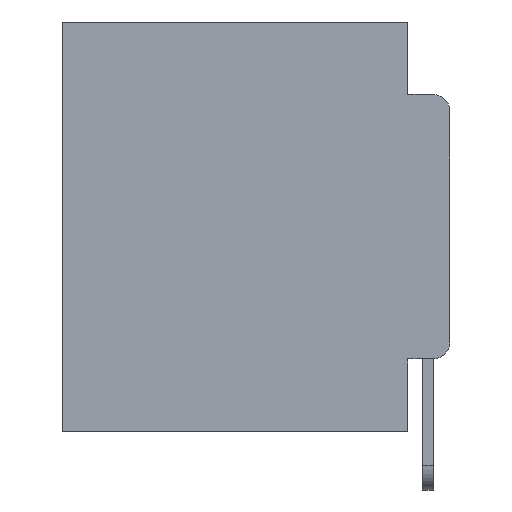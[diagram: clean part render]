
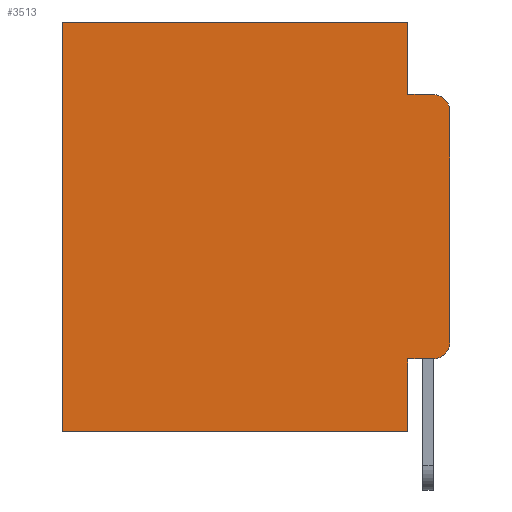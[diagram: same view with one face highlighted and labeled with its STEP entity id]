
A CAD part, left-side view. The second image highlights one B-rep face of the part: STEP entity #3513.
In plain terms, the highlighted planar face has unit normal (-1, 0, 0).
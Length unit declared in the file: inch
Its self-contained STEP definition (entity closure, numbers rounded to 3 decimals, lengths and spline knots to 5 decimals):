
#611 = EDGE_CURVE ( 'NONE', #26364, #8648, #3214, .T. ) ;
#617 = CARTESIAN_POINT ( 'NONE',  ( 0.298, 0., 0. ) ) ;
#1096 = CARTESIAN_POINT ( 'NONE',  ( 0.298, 0.473, 0. ) ) ;
#1326 = CARTESIAN_POINT ( 'NONE',  ( 0.298, 0., -0.1085 ) ) ;
#1452 = ORIENTED_EDGE ( 'NONE', *, *, #611, .F. ) ;
#1643 = CARTESIAN_POINT ( 'NONE',  ( 0.298, 0.051, -0.0885 ) ) ;
#1848 = CARTESIAN_POINT ( 'NONE',  ( 0.298, 0.051, -0.0885 ) ) ;
#2389 = CARTESIAN_POINT ( 'NONE',  ( 0.298, 0.473, 0. ) ) ;
#2427 = VECTOR ( 'NONE', #3080, 39.37008 ) ;
#2431 = DIRECTION ( 'NONE',  ( 0., 0., -1. ) ) ;
#2499 = VECTOR ( 'NONE', #6045, 39.37008 ) ;
#2696 = DIRECTION ( 'NONE',  ( -1., 0., 0. ) ) ;
#2914 = ORIENTED_EDGE ( 'NONE', *, *, #5883, .T. ) ;
#3080 = DIRECTION ( 'NONE',  ( 0., 1., 0. ) ) ;
#3214 = LINE ( 'NONE', #8234, #2499 ) ;
#3513 = ADVANCED_FACE ( 'NONE', ( #10835 ), #6703, .F. ) ;
#3762 = CARTESIAN_POINT ( 'NONE',  ( 0.298, 0.051, 0. ) ) ;
#3845 = DIRECTION ( 'NONE',  ( -1., 0., 0. ) ) ;
#5112 = CARTESIAN_POINT ( 'NONE',  ( 0.298, 0.473, -0.5 ) ) ;
#5298 = ORIENTED_EDGE ( 'NONE', *, *, #19797, .T. ) ;
#5883 = EDGE_CURVE ( 'NONE', #10238, #25235, #17625, .T. ) ;
#5884 = DIRECTION ( 'NONE',  ( 0., -1., 0. ) ) ;
#5976 = VECTOR ( 'NONE', #13088, 39.37008 ) ;
#5990 = VECTOR ( 'NONE', #16363, 39.37008 ) ;
#6045 = DIRECTION ( 'NONE',  ( 0., 0., -1. ) ) ;
#6703 = PLANE ( 'NONE',  #14835 ) ;
#6933 = ORIENTED_EDGE ( 'NONE', *, *, #10158, .F. ) ;
#7173 = CIRCLE ( 'NONE', #7552, 0.02 ) ;
#7238 = EDGE_CURVE ( 'NONE', #23879, #8241, #22629, .T. ) ;
#7552 = AXIS2_PLACEMENT_3D ( 'NONE', #15513, #2696, #17608 ) ;
#8087 = VERTEX_POINT ( 'NONE', #5112 ) ;
#8234 = CARTESIAN_POINT ( 'NONE',  ( 0.298, 0.051, 0. ) ) ;
#8241 = VERTEX_POINT ( 'NONE', #23570 ) ;
#8648 = VERTEX_POINT ( 'NONE', #22765 ) ;
#8827 = CARTESIAN_POINT ( 'NONE',  ( 0.298, 0., -0.3915 ) ) ;
#9230 = EDGE_CURVE ( 'NONE', #10996, #25235, #27058, .T. ) ;
#9503 = LINE ( 'NONE', #617, #2427 ) ;
#9953 = EDGE_CURVE ( 'NONE', #17269, #18759, #9503, .T. ) ;
#10158 = EDGE_CURVE ( 'NONE', #17269, #23879, #19641, .T. ) ;
#10238 = VERTEX_POINT ( 'NONE', #15059 ) ;
#10622 = ORIENTED_EDGE ( 'NONE', *, *, #9230, .F. ) ;
#10835 = FACE_OUTER_BOUND ( 'NONE', #18939, .T. ) ;
#10962 = ORIENTED_EDGE ( 'NONE', *, *, #11163, .F. ) ;
#10996 = VERTEX_POINT ( 'NONE', #1326 ) ;
#11163 = EDGE_CURVE ( 'NONE', #8648, #8087, #21993, .T. ) ;
#11412 = EDGE_CURVE ( 'NONE', #26364, #10238, #15588, .T. ) ;
#11514 = VECTOR ( 'NONE', #2431, 39.37008 ) ;
#12990 = ORIENTED_EDGE ( 'NONE', *, *, #11412, .T. ) ;
#13088 = DIRECTION ( 'NONE',  ( 0., 1., 0. ) ) ;
#14433 = DIRECTION ( 'NONE',  ( 0., 0., -1. ) ) ;
#14835 = AXIS2_PLACEMENT_3D ( 'NONE', #17648, #17606, #17929 ) ;
#15059 = CARTESIAN_POINT ( 'NONE',  ( 0.298, 0.02, -0.4115 ) ) ;
#15291 = CARTESIAN_POINT ( 'NONE',  ( 0.298, 0., 0. ) ) ;
#15295 = ORIENTED_EDGE ( 'NONE', *, *, #9953, .T. ) ;
#15513 = CARTESIAN_POINT ( 'NONE',  ( 0.298, 0.02, -0.1085 ) ) ;
#15588 = LINE ( 'NONE', #18509, #26225 ) ;
#16363 = DIRECTION ( 'NONE',  ( 0., -1., 0. ) ) ;
#16585 = DIRECTION ( 'NONE',  ( 0., 0., -1. ) ) ;
#16615 = CARTESIAN_POINT ( 'NONE',  ( 0.298, 0.051, 0. ) ) ;
#17269 = VERTEX_POINT ( 'NONE', #16615 ) ;
#17545 = ORIENTED_EDGE ( 'NONE', *, *, #7238, .F. ) ;
#17606 = DIRECTION ( 'NONE',  ( 1., 0., 0. ) ) ;
#17608 = DIRECTION ( 'NONE',  ( 0., 0., -1. ) ) ;
#17625 = CIRCLE ( 'NONE', #20854, 0.02 ) ;
#17648 = CARTESIAN_POINT ( 'NONE',  ( 0.298, 0., 0. ) ) ;
#17873 = CARTESIAN_POINT ( 'NONE',  ( 0.298, 0.051, -0.4115 ) ) ;
#17929 = DIRECTION ( 'NONE',  ( 0., 0., -1. ) ) ;
#18509 = CARTESIAN_POINT ( 'NONE',  ( 0.298, 0.051, -0.4115 ) ) ;
#18613 = CARTESIAN_POINT ( 'NONE',  ( 0.298, 0.02, -0.3915 ) ) ;
#18759 = VERTEX_POINT ( 'NONE', #2389 ) ;
#18939 = EDGE_LOOP ( 'NONE', ( #10622, #26847, #17545, #6933, #15295, #5298, #10962, #1452, #12990, #2914 ) ) ;
#19641 = LINE ( 'NONE', #3762, #24914 ) ;
#19797 = EDGE_CURVE ( 'NONE', #18759, #8087, #26965, .T. ) ;
#20854 = AXIS2_PLACEMENT_3D ( 'NONE', #18613, #3845, #16585 ) ;
#21782 = VECTOR ( 'NONE', #26049, 39.37008 ) ;
#21993 = LINE ( 'NONE', #25184, #5976 ) ;
#22629 = LINE ( 'NONE', #1848, #5990 ) ;
#22765 = CARTESIAN_POINT ( 'NONE',  ( 0.298, 0.051, -0.5 ) ) ;
#23570 = CARTESIAN_POINT ( 'NONE',  ( 0.298, 0.02, -0.0885 ) ) ;
#23879 = VERTEX_POINT ( 'NONE', #1643 ) ;
#24914 = VECTOR ( 'NONE', #14433, 39.37008 ) ;
#25184 = CARTESIAN_POINT ( 'NONE',  ( 0.298, 0., -0.5 ) ) ;
#25235 = VERTEX_POINT ( 'NONE', #8827 ) ;
#26049 = DIRECTION ( 'NONE',  ( 0., 0., -1. ) ) ;
#26213 = EDGE_CURVE ( 'NONE', #10996, #8241, #7173, .T. ) ;
#26225 = VECTOR ( 'NONE', #5884, 39.37008 ) ;
#26364 = VERTEX_POINT ( 'NONE', #17873 ) ;
#26847 = ORIENTED_EDGE ( 'NONE', *, *, #26213, .T. ) ;
#26965 = LINE ( 'NONE', #1096, #21782 ) ;
#27058 = LINE ( 'NONE', #15291, #11514 ) ;
